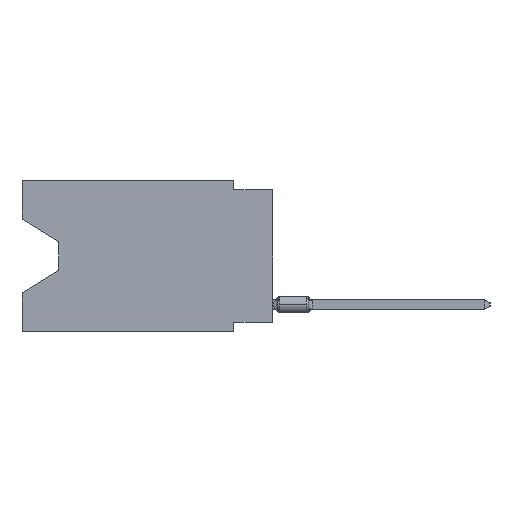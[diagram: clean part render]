
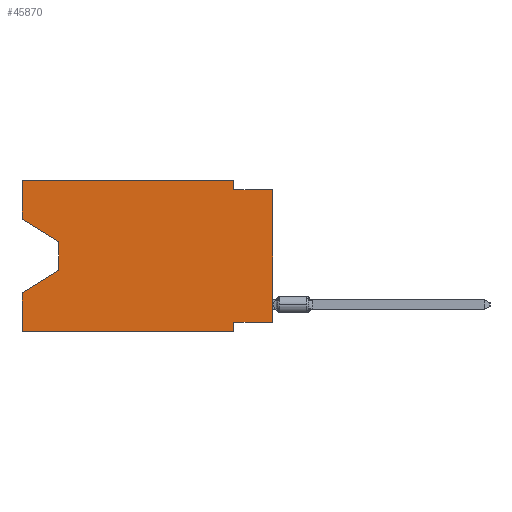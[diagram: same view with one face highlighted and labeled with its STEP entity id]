
A CAD part, left-side view. The second image highlights one B-rep face of the part: STEP entity #45870.
In plain terms, the highlighted planar face has unit normal (-1, 0, 0).
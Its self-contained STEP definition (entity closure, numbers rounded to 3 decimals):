
#1668 = CARTESIAN_POINT ( 'NONE',  ( 0., 13.97, -5.893 ) ) ;
#1761 = VERTEX_POINT ( 'NONE', #20151 ) ;
#3826 = VECTOR ( 'NONE', #34260, 1000. ) ;
#3903 = LINE ( 'NONE', #45601, #63716 ) ;
#4214 = DIRECTION ( 'NONE',  ( 0., 0., -1. ) ) ;
#5575 = CARTESIAN_POINT ( 'NONE',  ( 0., 0., -9.271 ) ) ;
#6176 = VERTEX_POINT ( 'NONE', #1668 ) ;
#7312 = LINE ( 'NONE', #58579, #53474 ) ;
#7626 = CARTESIAN_POINT ( 'NONE',  ( 0., 0., -9.271 ) ) ;
#7671 = CARTESIAN_POINT ( 'NONE',  ( 0., 0., 0. ) ) ;
#7989 = VERTEX_POINT ( 'NONE', #13303 ) ;
#9041 = LINE ( 'NONE', #40137, #48810 ) ;
#9186 = VECTOR ( 'NONE', #20798, 1000. ) ;
#9594 = CARTESIAN_POINT ( 'NONE',  ( 0., 16.383, -9.906 ) ) ;
#9631 = CARTESIAN_POINT ( 'NONE',  ( 0., 16.383, -9.906 ) ) ;
#9890 = VECTOR ( 'NONE', #64368, 1000. ) ;
#10700 = LINE ( 'NONE', #25414, #44508 ) ;
#12367 = EDGE_CURVE ( 'NONE', #52987, #18850, #24718, .T. ) ;
#12966 = DIRECTION ( 'NONE',  ( 0., -1., 0. ) ) ;
#13131 = DIRECTION ( 'NONE',  ( 0., 0., 1. ) ) ;
#13303 = CARTESIAN_POINT ( 'NONE',  ( 0., 16.383, 0. ) ) ;
#13450 = ORIENTED_EDGE ( 'NONE', *, *, #41551, .T. ) ;
#15121 = CARTESIAN_POINT ( 'NONE',  ( 0., 2.54, -9.906 ) ) ;
#15796 = DIRECTION ( 'NONE',  ( 0., 0., 1. ) ) ;
#16182 = ORIENTED_EDGE ( 'NONE', *, *, #47897, .F. ) ;
#16569 = VERTEX_POINT ( 'NONE', #35787 ) ;
#16785 = ORIENTED_EDGE ( 'NONE', *, *, #54972, .T. ) ;
#17005 = VERTEX_POINT ( 'NONE', #15121 ) ;
#18344 = LINE ( 'NONE', #60038, #34285 ) ;
#18850 = VERTEX_POINT ( 'NONE', #24190 ) ;
#18886 = EDGE_CURVE ( 'NONE', #45150, #18850, #30324, .T. ) ;
#19479 = ORIENTED_EDGE ( 'NONE', *, *, #63382, .F. ) ;
#20151 = CARTESIAN_POINT ( 'NONE',  ( 0., 16.383, -7.36 ) ) ;
#20798 = DIRECTION ( 'NONE',  ( 0., 0., -1. ) ) ;
#21108 = ORIENTED_EDGE ( 'NONE', *, *, #12367, .T. ) ;
#22363 = DIRECTION ( 'NONE',  ( 0., 0., -1. ) ) ;
#23717 = FACE_OUTER_BOUND ( 'NONE', #53884, .T. ) ;
#24190 = CARTESIAN_POINT ( 'NONE',  ( 0., 0., -0.635 ) ) ;
#24718 = LINE ( 'NONE', #7671, #49760 ) ;
#25018 = VECTOR ( 'NONE', #15796, 1000. ) ;
#25414 = CARTESIAN_POINT ( 'NONE',  ( 0., 16.383, 0. ) ) ;
#26073 = CARTESIAN_POINT ( 'NONE',  ( 0., 16.383, -2.546 ) ) ;
#28194 = AXIS2_PLACEMENT_3D ( 'NONE', #44561, #51039, #4214 ) ;
#28914 = DIRECTION ( 'NONE',  ( 0., 0., -1. ) ) ;
#30180 = PLANE ( 'NONE',  #28194 ) ;
#30324 = LINE ( 'NONE', #40244, #63452 ) ;
#31499 = LINE ( 'NONE', #41753, #25018 ) ;
#32376 = ORIENTED_EDGE ( 'NONE', *, *, #61613, .T. ) ;
#32921 = LINE ( 'NONE', #7626, #9890 ) ;
#33833 = ORIENTED_EDGE ( 'NONE', *, *, #64174, .T. ) ;
#34154 = LINE ( 'NONE', #65932, #34269 ) ;
#34260 = DIRECTION ( 'NONE',  ( 0., -1., 0. ) ) ;
#34269 = VECTOR ( 'NONE', #12966, 1000. ) ;
#34285 = VECTOR ( 'NONE', #28914, 1000. ) ;
#34829 = CARTESIAN_POINT ( 'NONE',  ( 0., 2.54, 0. ) ) ;
#34975 = ORIENTED_EDGE ( 'NONE', *, *, #54049, .F. ) ;
#35787 = CARTESIAN_POINT ( 'NONE',  ( 0., 13.97, -4.013 ) ) ;
#36383 = ORIENTED_EDGE ( 'NONE', *, *, #18886, .F. ) ;
#37647 = ORIENTED_EDGE ( 'NONE', *, *, #53694, .F. ) ;
#40137 = CARTESIAN_POINT ( 'NONE',  ( 0., 16.383, -2.546 ) ) ;
#40244 = CARTESIAN_POINT ( 'NONE',  ( 0., 0., -0.635 ) ) ;
#41551 = EDGE_CURVE ( 'NONE', #6176, #1761, #3903, .T. ) ;
#41753 = CARTESIAN_POINT ( 'NONE',  ( 0., 16.383, 0. ) ) ;
#41875 = EDGE_CURVE ( 'NONE', #60872, #45150, #18344, .T. ) ;
#42994 = LINE ( 'NONE', #58707, #9186 ) ;
#44145 = ORIENTED_EDGE ( 'NONE', *, *, #45234, .F. ) ;
#44508 = VECTOR ( 'NONE', #62315, 1000. ) ;
#44561 = CARTESIAN_POINT ( 'NONE',  ( 0., 16.383, 0. ) ) ;
#45150 = VERTEX_POINT ( 'NONE', #57198 ) ;
#45234 = EDGE_CURVE ( 'NONE', #58878, #7989, #10700, .T. ) ;
#45601 = CARTESIAN_POINT ( 'NONE',  ( 0., 13.97, -5.893 ) ) ;
#45870 = ADVANCED_FACE ( 'NONE', ( #23717 ), #30180, .F. ) ;
#46736 = DIRECTION ( 'NONE',  ( 0., -1., 0. ) ) ;
#47897 = EDGE_CURVE ( 'NONE', #52987, #66622, #32921, .T. ) ;
#48278 = ORIENTED_EDGE ( 'NONE', *, *, #41875, .F. ) ;
#48810 = VECTOR ( 'NONE', #60984, 1000. ) ;
#49760 = VECTOR ( 'NONE', #13131, 1000. ) ;
#49947 = CARTESIAN_POINT ( 'NONE',  ( 0., 2.54, -9.271 ) ) ;
#50390 = DIRECTION ( 'NONE',  ( 0., 0.855, -0.519 ) ) ;
#51039 = DIRECTION ( 'NONE',  ( 1., 0., 0. ) ) ;
#52987 = VERTEX_POINT ( 'NONE', #5575 ) ;
#53336 = VERTEX_POINT ( 'NONE', #9594 ) ;
#53474 = VECTOR ( 'NONE', #22363, 1000. ) ;
#53694 = EDGE_CURVE ( 'NONE', #7989, #60872, #34154, .T. ) ;
#53884 = EDGE_LOOP ( 'NONE', ( #32376, #33833, #13450, #19479, #16785, #34975, #16182, #21108, #36383, #48278, #37647, #44145 ) ) ;
#54049 = EDGE_CURVE ( 'NONE', #66622, #17005, #42994, .T. ) ;
#54972 = EDGE_CURVE ( 'NONE', #53336, #17005, #65361, .T. ) ;
#57198 = CARTESIAN_POINT ( 'NONE',  ( 0., 2.54, -0.635 ) ) ;
#58579 = CARTESIAN_POINT ( 'NONE',  ( 0., 13.97, -4.013 ) ) ;
#58707 = CARTESIAN_POINT ( 'NONE',  ( 0., 2.54, -9.906 ) ) ;
#58878 = VERTEX_POINT ( 'NONE', #26073 ) ;
#60038 = CARTESIAN_POINT ( 'NONE',  ( 0., 2.54, 0. ) ) ;
#60872 = VERTEX_POINT ( 'NONE', #34829 ) ;
#60984 = DIRECTION ( 'NONE',  ( 0., -0.855, -0.519 ) ) ;
#61613 = EDGE_CURVE ( 'NONE', #58878, #16569, #9041, .T. ) ;
#62315 = DIRECTION ( 'NONE',  ( 0., 0., 1. ) ) ;
#63382 = EDGE_CURVE ( 'NONE', #53336, #1761, #31499, .T. ) ;
#63452 = VECTOR ( 'NONE', #46736, 1000. ) ;
#63716 = VECTOR ( 'NONE', #50390, 1000. ) ;
#64174 = EDGE_CURVE ( 'NONE', #16569, #6176, #7312, .T. ) ;
#64368 = DIRECTION ( 'NONE',  ( 0., 1., 0. ) ) ;
#65361 = LINE ( 'NONE', #9631, #3826 ) ;
#65932 = CARTESIAN_POINT ( 'NONE',  ( 0., 16.383, 0. ) ) ;
#66622 = VERTEX_POINT ( 'NONE', #49947 ) ;
